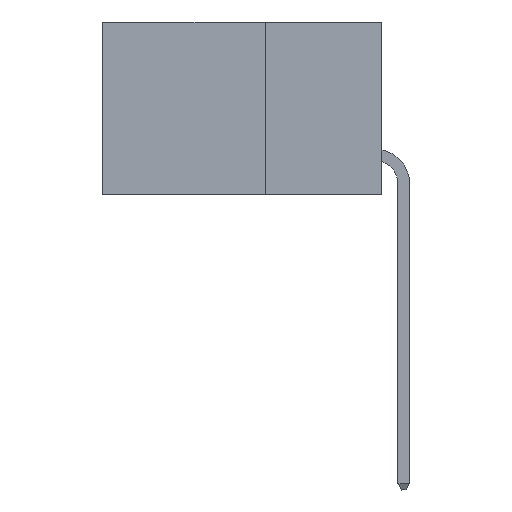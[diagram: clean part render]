
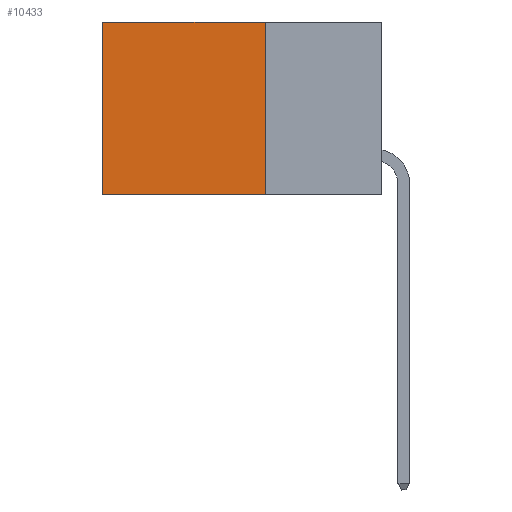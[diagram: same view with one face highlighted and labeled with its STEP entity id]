
A CAD part, left-side view. The second image highlights one B-rep face of the part: STEP entity #10433.
In plain terms, the highlighted planar face has unit normal (-1, 0, 0).
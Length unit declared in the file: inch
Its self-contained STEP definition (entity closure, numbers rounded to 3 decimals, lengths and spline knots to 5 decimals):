
#85 = AXIS2_PLACEMENT_3D ( 'NONE', #9476, #16898, #16706 ) ;
#587 = CARTESIAN_POINT ( 'NONE',  ( 0.2875, 0.6, 0. ) ) ;
#1140 = LINE ( 'NONE', #9053, #15077 ) ;
#1496 = ORIENTED_EDGE ( 'NONE', *, *, #9833, .F. ) ;
#1719 = DIRECTION ( 'NONE',  ( 0., 1., 0. ) ) ;
#2166 = VERTEX_POINT ( 'NONE', #587 ) ;
#2358 = ORIENTED_EDGE ( 'NONE', *, *, #8383, .T. ) ;
#2830 = CARTESIAN_POINT ( 'NONE',  ( 0.2875, 0.25, 0. ) ) ;
#2965 = DIRECTION ( 'NONE',  ( 0., 1., 0. ) ) ;
#4549 = CARTESIAN_POINT ( 'NONE',  ( 0.2875, 0.25, 0. ) ) ;
#6860 = EDGE_LOOP ( 'NONE', ( #2358, #16002, #1496, #18676 ) ) ;
#7892 = CARTESIAN_POINT ( 'NONE',  ( 0.2875, 0.25, -0.37 ) ) ;
#8383 = EDGE_CURVE ( 'NONE', #2166, #14851, #10989, .T. ) ;
#8852 = LINE ( 'NONE', #7892, #10509 ) ;
#9053 = CARTESIAN_POINT ( 'NONE',  ( 0.2875, 0.25, 0. ) ) ;
#9118 = DIRECTION ( 'NONE',  ( 0., 0., -1. ) ) ;
#9296 = EDGE_CURVE ( 'NONE', #12493, #2166, #9993, .T. ) ;
#9476 = CARTESIAN_POINT ( 'NONE',  ( 0.2875, 0.25, 0. ) ) ;
#9833 = EDGE_CURVE ( 'NONE', #12493, #16569, #1140, .T. ) ;
#9993 = LINE ( 'NONE', #2830, #16728 ) ;
#10433 = ADVANCED_FACE ( 'NONE', ( #17158 ), #13906, .F. ) ;
#10509 = VECTOR ( 'NONE', #1719, 39.37008 ) ;
#10680 = CARTESIAN_POINT ( 'NONE',  ( 0.2875, 0.6, 0. ) ) ;
#10989 = LINE ( 'NONE', #10680, #16079 ) ;
#12493 = VERTEX_POINT ( 'NONE', #4549 ) ;
#13252 = CARTESIAN_POINT ( 'NONE',  ( 0.2875, 0.25, -0.37 ) ) ;
#13906 = PLANE ( 'NONE',  #85 ) ;
#14851 = VERTEX_POINT ( 'NONE', #17099 ) ;
#15077 = VECTOR ( 'NONE', #9118, 39.37008 ) ;
#16002 = ORIENTED_EDGE ( 'NONE', *, *, #16239, .F. ) ;
#16079 = VECTOR ( 'NONE', #18248, 39.37008 ) ;
#16239 = EDGE_CURVE ( 'NONE', #16569, #14851, #8852, .T. ) ;
#16569 = VERTEX_POINT ( 'NONE', #13252 ) ;
#16706 = DIRECTION ( 'NONE',  ( 0., 0., -1. ) ) ;
#16728 = VECTOR ( 'NONE', #2965, 39.37008 ) ;
#16898 = DIRECTION ( 'NONE',  ( 1., 0., 0. ) ) ;
#17099 = CARTESIAN_POINT ( 'NONE',  ( 0.2875, 0.6, -0.37 ) ) ;
#17158 = FACE_OUTER_BOUND ( 'NONE', #6860, .T. ) ;
#18248 = DIRECTION ( 'NONE',  ( 0., 0., -1. ) ) ;
#18676 = ORIENTED_EDGE ( 'NONE', *, *, #9296, .T. ) ;
